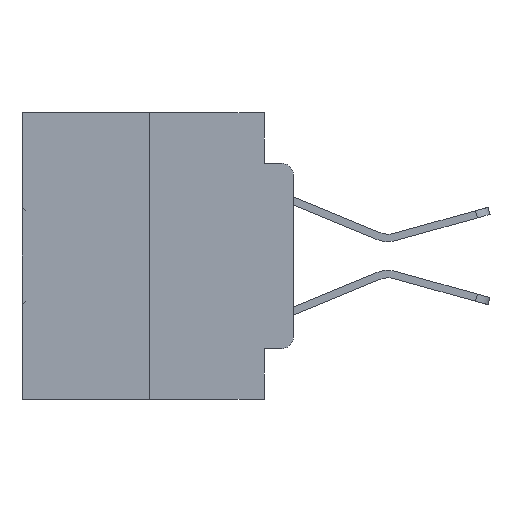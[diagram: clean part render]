
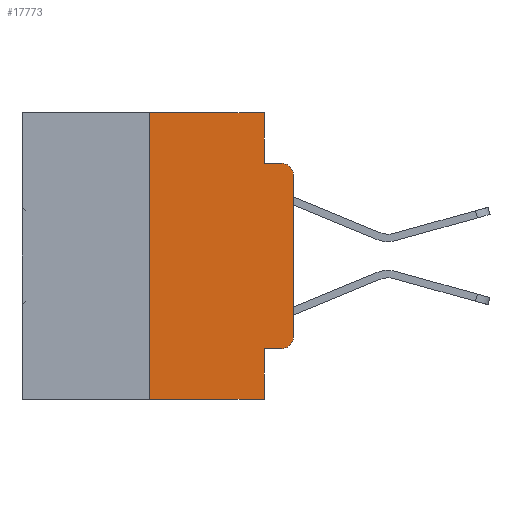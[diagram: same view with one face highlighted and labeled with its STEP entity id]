
A CAD part, left-side view. The second image highlights one B-rep face of the part: STEP entity #17773.
In plain terms, the highlighted planar face has unit normal (-1, 0, 0).
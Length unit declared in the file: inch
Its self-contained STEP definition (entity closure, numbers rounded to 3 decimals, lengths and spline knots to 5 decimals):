
#529 = ORIENTED_EDGE ( 'NONE', *, *, #14978, .F. ) ;
#893 = ORIENTED_EDGE ( 'NONE', *, *, #14399, .T. ) ;
#1028 = CARTESIAN_POINT ( 'NONE',  ( 0., 0.051, -0.4115 ) ) ;
#1047 = VECTOR ( 'NONE', #7452, 39.37008 ) ;
#1689 = CARTESIAN_POINT ( 'NONE',  ( 0., 0.02, -0.4115 ) ) ;
#1933 = ORIENTED_EDGE ( 'NONE', *, *, #12276, .F. ) ;
#2109 = ORIENTED_EDGE ( 'NONE', *, *, #14346, .T. ) ;
#2427 = DIRECTION ( 'NONE',  ( 0., -1., 0. ) ) ;
#3250 = LINE ( 'NONE', #10902, #10915 ) ;
#3430 = FACE_OUTER_BOUND ( 'NONE', #16000, .T. ) ;
#3956 = ORIENTED_EDGE ( 'NONE', *, *, #24912, .T. ) ;
#4181 = CARTESIAN_POINT ( 'NONE',  ( 0., 0.473, 0. ) ) ;
#4262 = ORIENTED_EDGE ( 'NONE', *, *, #31387, .F. ) ;
#5222 = AXIS2_PLACEMENT_3D ( 'NONE', #15181, #32317, #17743 ) ;
#6786 = PLANE ( 'NONE',  #11913 ) ;
#7235 = CARTESIAN_POINT ( 'NONE',  ( 0., 0., -0.1085 ) ) ;
#7452 = DIRECTION ( 'NONE',  ( 0., 0., -1. ) ) ;
#7744 = AXIS2_PLACEMENT_3D ( 'NONE', #13823, #30956, #16319 ) ;
#7781 = ORIENTED_EDGE ( 'NONE', *, *, #26104, .T. ) ;
#7985 = CARTESIAN_POINT ( 'NONE',  ( 0., 0.25, 0. ) ) ;
#8753 = VERTEX_POINT ( 'NONE', #12380 ) ;
#9330 = DIRECTION ( 'NONE',  ( 1., 0., 0. ) ) ;
#10391 = VERTEX_POINT ( 'NONE', #28726 ) ;
#10902 = CARTESIAN_POINT ( 'NONE',  ( 0., 0.473, -0.5 ) ) ;
#10915 = VECTOR ( 'NONE', #28145, 39.37008 ) ;
#11325 = CARTESIAN_POINT ( 'NONE',  ( 0., 0.051, 0. ) ) ;
#11815 = VERTEX_POINT ( 'NONE', #15988 ) ;
#11913 = AXIS2_PLACEMENT_3D ( 'NONE', #4181, #9330, #26656 ) ;
#11975 = ORIENTED_EDGE ( 'NONE', *, *, #13326, .F. ) ;
#12065 = VECTOR ( 'NONE', #27787, 39.37008 ) ;
#12276 = EDGE_CURVE ( 'NONE', #8753, #11815, #25981, .T. ) ;
#12380 = CARTESIAN_POINT ( 'NONE',  ( 0., 0.051, -0.4115 ) ) ;
#12726 = DIRECTION ( 'NONE',  ( 0., 0., -1. ) ) ;
#13038 = VERTEX_POINT ( 'NONE', #11325 ) ;
#13113 = CARTESIAN_POINT ( 'NONE',  ( 0., 0., -0.3915 ) ) ;
#13326 = EDGE_CURVE ( 'NONE', #13038, #10391, #28560, .T. ) ;
#13823 = CARTESIAN_POINT ( 'NONE',  ( 0., 0.02, -0.3915 ) ) ;
#14346 = EDGE_CURVE ( 'NONE', #23680, #23497, #24116, .T. ) ;
#14399 = EDGE_CURVE ( 'NONE', #23987, #11815, #3250, .T. ) ;
#14456 = CIRCLE ( 'NONE', #5222, 0.02 ) ;
#14900 = VECTOR ( 'NONE', #26269, 39.37008 ) ;
#14978 = EDGE_CURVE ( 'NONE', #23987, #19434, #19491, .T. ) ;
#15016 = LINE ( 'NONE', #32309, #26561 ) ;
#15133 = DIRECTION ( 'NONE',  ( 0., -1., 0. ) ) ;
#15181 = CARTESIAN_POINT ( 'NONE',  ( 0., 0.02, -0.1085 ) ) ;
#15462 = CARTESIAN_POINT ( 'NONE',  ( 0., 0.02, -0.0885 ) ) ;
#15698 = CARTESIAN_POINT ( 'NONE',  ( 0., 0.25, 0. ) ) ;
#15709 = DIRECTION ( 'NONE',  ( 0., 0., 1. ) ) ;
#15988 = CARTESIAN_POINT ( 'NONE',  ( 0., 0.051, -0.5 ) ) ;
#16000 = EDGE_LOOP ( 'NONE', ( #2109, #3956, #4262, #11975, #16824, #529, #893, #1933, #18564, #7781 ) ) ;
#16319 = DIRECTION ( 'NONE',  ( 0., 0., -1. ) ) ;
#16704 = CIRCLE ( 'NONE', #7744, 0.02 ) ;
#16824 = ORIENTED_EDGE ( 'NONE', *, *, #27617, .F. ) ;
#17456 = CARTESIAN_POINT ( 'NONE',  ( 0., 0.051, 0. ) ) ;
#17743 = DIRECTION ( 'NONE',  ( 0., 0., -1. ) ) ;
#17773 = ADVANCED_FACE ( 'NONE', ( #3430 ), #6786, .F. ) ;
#18564 = ORIENTED_EDGE ( 'NONE', *, *, #18962, .T. ) ;
#18697 = VECTOR ( 'NONE', #15709, 39.37008 ) ;
#18741 = VECTOR ( 'NONE', #12726, 39.37008 ) ;
#18962 = EDGE_CURVE ( 'NONE', #8753, #29121, #21525, .T. ) ;
#19434 = VERTEX_POINT ( 'NONE', #15698 ) ;
#19491 = LINE ( 'NONE', #7985, #12065 ) ;
#21525 = LINE ( 'NONE', #1028, #14900 ) ;
#21670 = CARTESIAN_POINT ( 'NONE',  ( 0., 0.25, -0.5 ) ) ;
#23497 = VERTEX_POINT ( 'NONE', #7235 ) ;
#23680 = VERTEX_POINT ( 'NONE', #13113 ) ;
#23987 = VERTEX_POINT ( 'NONE', #21670 ) ;
#24116 = LINE ( 'NONE', #30371, #18697 ) ;
#24604 = VECTOR ( 'NONE', #15133, 39.37008 ) ;
#24912 = EDGE_CURVE ( 'NONE', #23497, #32003, #14456, .T. ) ;
#25981 = LINE ( 'NONE', #29897, #18741 ) ;
#26104 = EDGE_CURVE ( 'NONE', #29121, #23680, #16704, .T. ) ;
#26269 = DIRECTION ( 'NONE',  ( 0., -1., 0. ) ) ;
#26561 = VECTOR ( 'NONE', #2427, 39.37008 ) ;
#26656 = DIRECTION ( 'NONE',  ( 0., 0., -1. ) ) ;
#27389 = CARTESIAN_POINT ( 'NONE',  ( 0., 0.473, 0. ) ) ;
#27617 = EDGE_CURVE ( 'NONE', #19434, #13038, #31020, .T. ) ;
#27787 = DIRECTION ( 'NONE',  ( 0., 0., 1. ) ) ;
#28145 = DIRECTION ( 'NONE',  ( 0., -1., 0. ) ) ;
#28560 = LINE ( 'NONE', #17456, #1047 ) ;
#28726 = CARTESIAN_POINT ( 'NONE',  ( 0., 0.051, -0.0885 ) ) ;
#29121 = VERTEX_POINT ( 'NONE', #1689 ) ;
#29897 = CARTESIAN_POINT ( 'NONE',  ( 0., 0.051, 0. ) ) ;
#30371 = CARTESIAN_POINT ( 'NONE',  ( 0., 0., 0. ) ) ;
#30956 = DIRECTION ( 'NONE',  ( -1., 0., 0. ) ) ;
#31020 = LINE ( 'NONE', #27389, #24604 ) ;
#31387 = EDGE_CURVE ( 'NONE', #10391, #32003, #15016, .T. ) ;
#32003 = VERTEX_POINT ( 'NONE', #15462 ) ;
#32309 = CARTESIAN_POINT ( 'NONE',  ( 0., 0.051, -0.0885 ) ) ;
#32317 = DIRECTION ( 'NONE',  ( -1., 0., 0. ) ) ;
